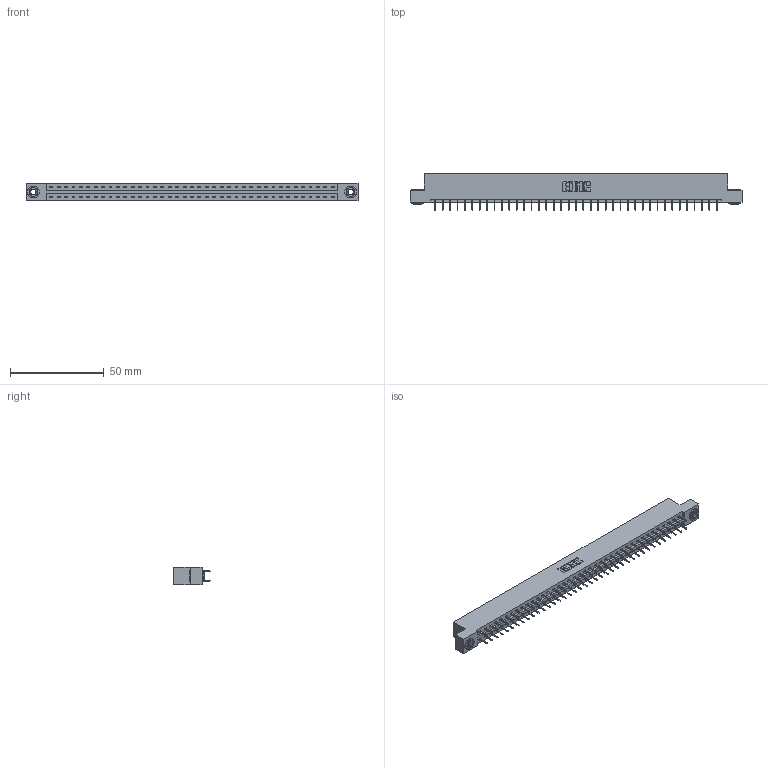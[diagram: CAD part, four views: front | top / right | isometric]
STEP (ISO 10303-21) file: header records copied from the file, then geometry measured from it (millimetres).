
FILE_DESCRIPTION (( 'STEP AP203' ), '1' );
FILE_NAME ('387-078-524-203.STEP', '2019-10-22T05:37:55', ( '' ), ( '' ), 'SwSTEP 2.0', 'SolidWorks 2016', '' );
FILE_SCHEMA (( 'CONFIG_CONTROL_DESIGN' ));
Length unit declared in the file: inch
Products named in the file (4): 387-078-524-203; 345-292-001_345-293-124; 337 Part_Flush Mounting Lugs - 0.156 Dia-TH; 345-250-002_345-250-002-102
Assembly tree (81 placements, depth 2):
  387-078-524-203
    337 Part_Flush Mounting Lugs - 0.156 Dia-TH
    345-292-001_345-293-124  x78
    345-250-002_345-250-002-102  x2
Bounding box: 177.55 x 19.69 x 9.4 mm (x, y, z)
Volume: 18572.6 mm3; surface area: 20826.1 mm2
Topology: 81 solids, 81 shells, 4676 faces, 13257 edges, 8522 vertices
Faces by surface type: plane 3512, cylinder 1156, cone 8
Entity records: 31350 total; most frequent: CARTESIAN_POINT 5257, ORIENTED_EDGE 5186, DIRECTION 4511, EDGE_CURVE 2593, VECTOR 2445, LINE 2445, VERTEX_POINT 1722, AXIS2_PLACEMENT_3D 1033
